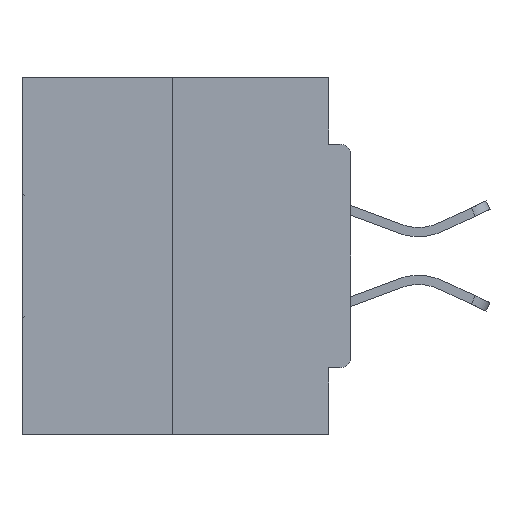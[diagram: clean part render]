
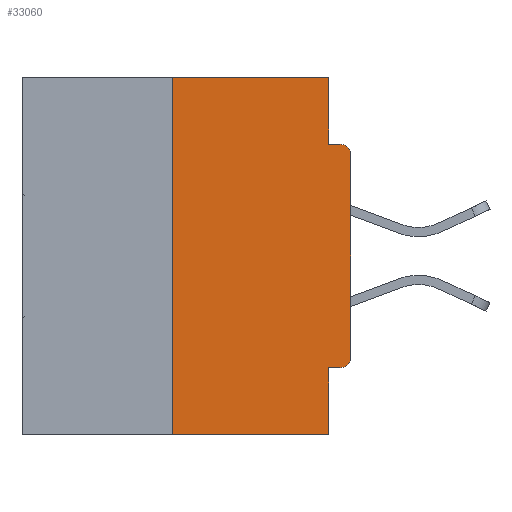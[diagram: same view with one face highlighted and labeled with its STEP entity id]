
A CAD part, left-side view. The second image highlights one B-rep face of the part: STEP entity #33060.
In plain terms, the highlighted planar face has unit normal (-1, 0, 0).
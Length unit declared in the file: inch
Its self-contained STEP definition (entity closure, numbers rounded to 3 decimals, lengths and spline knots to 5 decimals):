
#233 = VERTEX_POINT ( 'NONE', #2909 ) ;
#396 = ORIENTED_EDGE ( 'NONE', *, *, #30817, .F. ) ;
#1006 = VERTEX_POINT ( 'NONE', #19104 ) ;
#1342 = FACE_OUTER_BOUND ( 'NONE', #18859, .T. ) ;
#1365 = VECTOR ( 'NONE', #32677, 39.37008 ) ;
#1673 = ORIENTED_EDGE ( 'NONE', *, *, #37795, .F. ) ;
#2019 = EDGE_CURVE ( 'NONE', #9244, #32871, #10171, .T. ) ;
#2530 = VERTEX_POINT ( 'NONE', #26390 ) ;
#2690 = EDGE_CURVE ( 'NONE', #5433, #2530, #18570, .T. ) ;
#2909 = CARTESIAN_POINT ( 'NONE',  ( 0., 0.25, 0. ) ) ;
#3617 = VERTEX_POINT ( 'NONE', #27745 ) ;
#4202 = DIRECTION ( 'NONE',  ( 0., 0., -1. ) ) ;
#4252 = VERTEX_POINT ( 'NONE', #19659 ) ;
#4456 = CARTESIAN_POINT ( 'NONE',  ( 0., 0.25, 0. ) ) ;
#4672 = EDGE_CURVE ( 'NONE', #3617, #2530, #12948, .T. ) ;
#5109 = DIRECTION ( 'NONE',  ( 0., 0., -1. ) ) ;
#5433 = VERTEX_POINT ( 'NONE', #40273 ) ;
#6759 = VECTOR ( 'NONE', #5109, 39.37008 ) ;
#7031 = LINE ( 'NONE', #7859, #39663 ) ;
#7331 = DIRECTION ( 'NONE',  ( 0., 0., 1. ) ) ;
#7699 = CARTESIAN_POINT ( 'NONE',  ( 0., 0., -0.4065 ) ) ;
#7859 = CARTESIAN_POINT ( 'NONE',  ( 0., 0., 0. ) ) ;
#8259 = ORIENTED_EDGE ( 'NONE', *, *, #34110, .F. ) ;
#8552 = VECTOR ( 'NONE', #7331, 39.37008 ) ;
#9244 = VERTEX_POINT ( 'NONE', #32265 ) ;
#9632 = EDGE_CURVE ( 'NONE', #32871, #4252, #7031, .T. ) ;
#10171 = CIRCLE ( 'NONE', #35203, 0.015 ) ;
#10434 = DIRECTION ( 'NONE',  ( 0., 0., -1. ) ) ;
#10509 = VECTOR ( 'NONE', #23098, 39.37008 ) ;
#10559 = LINE ( 'NONE', #23250, #10509 ) ;
#11037 = DIRECTION ( 'NONE',  ( 0., 0., 1. ) ) ;
#11565 = CARTESIAN_POINT ( 'NONE',  ( 0., 0.031, -0.5 ) ) ;
#12091 = CARTESIAN_POINT ( 'NONE',  ( 0., 0.015, -0.1085 ) ) ;
#12136 = LINE ( 'NONE', #31999, #36379 ) ;
#12298 = CIRCLE ( 'NONE', #35024, 0.015 ) ;
#12948 = LINE ( 'NONE', #27812, #36732 ) ;
#13100 = DIRECTION ( 'NONE',  ( 1., 0., 0. ) ) ;
#14224 = CARTESIAN_POINT ( 'NONE',  ( 0., 0.015, -0.3915 ) ) ;
#14487 = ORIENTED_EDGE ( 'NONE', *, *, #2690, .F. ) ;
#16090 = EDGE_CURVE ( 'NONE', #4252, #1006, #12298, .T. ) ;
#17498 = EDGE_CURVE ( 'NONE', #39256, #1006, #29997, .T. ) ;
#17555 = CARTESIAN_POINT ( 'NONE',  ( 0., 0.031, -0.0935 ) ) ;
#18425 = DIRECTION ( 'NONE',  ( 0., 0., -1. ) ) ;
#18570 = LINE ( 'NONE', #11565, #6759 ) ;
#18859 = EDGE_LOOP ( 'NONE', ( #396, #26007, #20731, #14487, #8259, #22818, #33699, #34329, #20578, #1673 ) ) ;
#18914 = CARTESIAN_POINT ( 'NONE',  ( 0., 0.031, 0. ) ) ;
#19104 = CARTESIAN_POINT ( 'NONE',  ( 0., 0.015, -0.0935 ) ) ;
#19659 = CARTESIAN_POINT ( 'NONE',  ( 0., 0., -0.1085 ) ) ;
#20578 = ORIENTED_EDGE ( 'NONE', *, *, #17498, .F. ) ;
#20587 = DIRECTION ( 'NONE',  ( 0., 0., -1. ) ) ;
#20731 = ORIENTED_EDGE ( 'NONE', *, *, #4672, .T. ) ;
#21918 = DIRECTION ( 'NONE',  ( -1., 0., 0. ) ) ;
#21958 = VECTOR ( 'NONE', #36016, 39.37008 ) ;
#22550 = CARTESIAN_POINT ( 'NONE',  ( 0., 0.46, 0. ) ) ;
#22818 = ORIENTED_EDGE ( 'NONE', *, *, #2019, .T. ) ;
#22897 = CARTESIAN_POINT ( 'NONE',  ( 0., 0., -0.0935 ) ) ;
#23098 = DIRECTION ( 'NONE',  ( 0., -1., 0. ) ) ;
#23250 = CARTESIAN_POINT ( 'NONE',  ( 0., 0.46, 0. ) ) ;
#26007 = ORIENTED_EDGE ( 'NONE', *, *, #39388, .F. ) ;
#26390 = CARTESIAN_POINT ( 'NONE',  ( 0., 0.031, -0.5 ) ) ;
#27745 = CARTESIAN_POINT ( 'NONE',  ( 0., 0.25, -0.5 ) ) ;
#27812 = CARTESIAN_POINT ( 'NONE',  ( 0., 0.46, -0.5 ) ) ;
#28887 = LINE ( 'NONE', #7699, #21958 ) ;
#29997 = LINE ( 'NONE', #22897, #1365 ) ;
#30817 = EDGE_CURVE ( 'NONE', #233, #31550, #10559, .T. ) ;
#31550 = VERTEX_POINT ( 'NONE', #18914 ) ;
#31999 = CARTESIAN_POINT ( 'NONE',  ( 0., 0.031, 0. ) ) ;
#32199 = PLANE ( 'NONE',  #39401 ) ;
#32265 = CARTESIAN_POINT ( 'NONE',  ( 0., 0.015, -0.4065 ) ) ;
#32677 = DIRECTION ( 'NONE',  ( 0., -1., 0. ) ) ;
#32871 = VERTEX_POINT ( 'NONE', #34418 ) ;
#33060 = ADVANCED_FACE ( 'NONE', ( #1342 ), #32199, .F. ) ;
#33699 = ORIENTED_EDGE ( 'NONE', *, *, #9632, .T. ) ;
#33759 = LINE ( 'NONE', #4456, #8552 ) ;
#34110 = EDGE_CURVE ( 'NONE', #9244, #5433, #28887, .T. ) ;
#34329 = ORIENTED_EDGE ( 'NONE', *, *, #16090, .T. ) ;
#34418 = CARTESIAN_POINT ( 'NONE',  ( 0., 0., -0.3915 ) ) ;
#35024 = AXIS2_PLACEMENT_3D ( 'NONE', #12091, #21918, #18425 ) ;
#35203 = AXIS2_PLACEMENT_3D ( 'NONE', #14224, #36354, #20587 ) ;
#36016 = DIRECTION ( 'NONE',  ( 0., 1., 0. ) ) ;
#36354 = DIRECTION ( 'NONE',  ( -1., 0., 0. ) ) ;
#36379 = VECTOR ( 'NONE', #10434, 39.37008 ) ;
#36732 = VECTOR ( 'NONE', #40367, 39.37008 ) ;
#37795 = EDGE_CURVE ( 'NONE', #31550, #39256, #12136, .T. ) ;
#39256 = VERTEX_POINT ( 'NONE', #17555 ) ;
#39388 = EDGE_CURVE ( 'NONE', #3617, #233, #33759, .T. ) ;
#39401 = AXIS2_PLACEMENT_3D ( 'NONE', #22550, #13100, #4202 ) ;
#39663 = VECTOR ( 'NONE', #11037, 39.37008 ) ;
#40273 = CARTESIAN_POINT ( 'NONE',  ( 0., 0.031, -0.4065 ) ) ;
#40367 = DIRECTION ( 'NONE',  ( 0., -1., 0. ) ) ;
